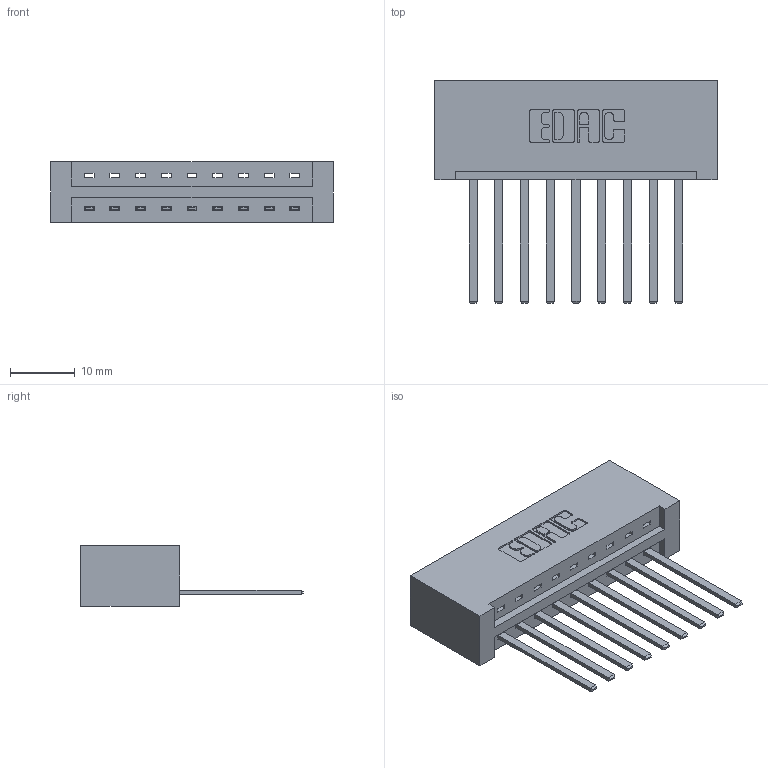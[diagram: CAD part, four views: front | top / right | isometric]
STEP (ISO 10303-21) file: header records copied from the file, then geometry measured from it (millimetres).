
FILE_DESCRIPTION (( 'STEP AP203' ), '1' );
FILE_NAME ('387-009-544-101.STEP', '2018-09-10T06:01:41', ( '' ), ( '' ), 'SwSTEP 2.0', 'SolidWorks 2016', '' );
FILE_SCHEMA (( 'CONFIG_CONTROL_DESIGN' ));
Length unit declared in the file: inch
Products named in the file (3): 337 Part_No Mounting Lugs; 345-292-001_345-293-144; 387-009-544-101
Assembly tree (10 placements, depth 2):
  387-009-544-101
    337 Part_No Mounting Lugs
    345-292-001_345-293-144  x9
Bounding box: 43.54 x 34.3 x 9.4 mm (x, y, z)
Volume: 4954.8 mm3; surface area: 5261.2 mm2
Topology: 10 solids, 10 shells, 610 faces, 1817 edges, 1198 vertices
Faces by surface type: plane 444, cylinder 166
Entity records: 10497 total; most frequent: CARTESIAN_POINT 1833, ORIENTED_EDGE 1778, DIRECTION 1599, EDGE_CURVE 889, VECTOR 773, LINE 773, VERTEX_POINT 590, AXIS2_PLACEMENT_3D 413
